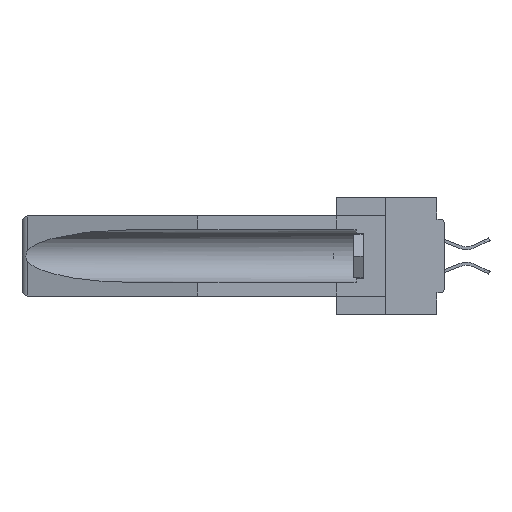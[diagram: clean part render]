
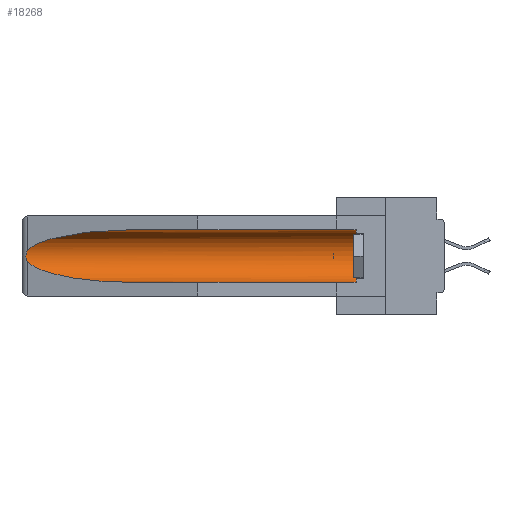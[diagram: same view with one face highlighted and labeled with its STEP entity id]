
A CAD part, left-side view. The second image highlights one B-rep face of the part: STEP entity #18268.
In plain terms, the highlighted cylindrical face has radius 2.857 mm (diameter 5.715 mm), a partial arc.
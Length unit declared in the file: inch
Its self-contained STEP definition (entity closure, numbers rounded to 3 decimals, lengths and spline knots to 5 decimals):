
#1574 =( BOUNDED_CURVE ( )  B_SPLINE_CURVE ( 3, ( #16158, #28046, #19972, #5374 ),
 .UNSPECIFIED., .F., .F. ) 
 B_SPLINE_CURVE_WITH_KNOTS ( ( 4, 4 ),
 ( 4.71239, 6.08839 ),
 .UNSPECIFIED. ) 
 CURVE ( )  GEOMETRIC_REPRESENTATION_ITEM ( )  RATIONAL_B_SPLINE_CURVE ( ( 1., 0.848, 0.848, 1. ) ) 
 REPRESENTATION_ITEM ( '' )  );
#3308 = CARTESIAN_POINT ( 'NONE',  ( 0.26597, 1.5296, -0.19026 ) ) ;
#5374 = CARTESIAN_POINT ( 'NONE',  ( 0.26537, 1.52718, -0.14972 ) ) ;
#6934 = LINE ( 'NONE', #43947, #14084 ) ;
#10229 = CYLINDRICAL_SURFACE ( 'NONE', #19563, 0.1125 ) ;
#10656 = CARTESIAN_POINT ( 'NONE',  ( 0.26537, 1.52718, -0.14972 ) ) ;
#10883 = CARTESIAN_POINT ( 'NONE',  ( 0.25451, 1.48313, -0.24835 ) ) ;
#11092 = CARTESIAN_POINT ( 'NONE',  ( 0.26655, 1.53094, -0.18657 ) ) ;
#12966 = CARTESIAN_POINT ( 'NONE',  ( 0.155, 1.07973, -0.284 ) ) ;
#14084 = VECTOR ( 'NONE', #48096, 39.37008 ) ;
#14113 = EDGE_CURVE ( 'NONE', #47181, #30268, #31578, .T. ) ;
#14117 = CARTESIAN_POINT ( 'NONE',  ( 0.26537, 1.52718, -0.19328 ) ) ;
#16128 = ORIENTED_EDGE ( 'NONE', *, *, #14113, .T. ) ;
#16158 = CARTESIAN_POINT ( 'NONE',  ( 0.155, 1.07973, -0.059 ) ) ;
#17837 = CARTESIAN_POINT ( 'NONE',  ( 0.26537, 1.52718, -0.14972 ) ) ;
#18268 = ADVANCED_FACE ( 'NONE', ( #47509 ), #10229, .F. ) ;
#18936 = VECTOR ( 'NONE', #21263, 39.37008 ) ;
#19563 = AXIS2_PLACEMENT_3D ( 'NONE', #37400, #22460, #33725 ) ;
#19953 = VERTEX_POINT ( 'NONE', #10656 ) ;
#19972 = CARTESIAN_POINT ( 'NONE',  ( 0.25451, 1.48313, -0.09465 ) ) ;
#20417 = CARTESIAN_POINT ( 'NONE',  ( 0.155, 1.07973, -0.059 ) ) ;
#20473 = CARTESIAN_POINT ( 'NONE',  ( 0.155, 0.126, -0.284 ) ) ;
#21263 = DIRECTION ( 'NONE',  ( 0., 1., 0. ) ) ;
#21449 = CARTESIAN_POINT ( 'NONE',  ( 0.26537, 1.52718, -0.19328 ) ) ;
#21588 = CARTESIAN_POINT ( 'NONE',  ( 0.155, -0.30754, -0.284 ) ) ;
#21740 = VERTEX_POINT ( 'NONE', #12966 ) ;
#22326 = CARTESIAN_POINT ( 'NONE',  ( 0.2675, 1.53308, -0.16763 ) ) ;
#22460 = DIRECTION ( 'NONE',  ( 0., 1., 0. ) ) ;
#22610 = EDGE_CURVE ( 'NONE', #37129, #19953, #1574, .T. ) ;
#26129 = CARTESIAN_POINT ( 'NONE',  ( 0.26537, 1.52718, -0.19328 ) ) ;
#26180 = CARTESIAN_POINT ( 'NONE',  ( 0.155, 0.126, -0.1715 ) ) ;
#26446 = CARTESIAN_POINT ( 'NONE',  ( 0.2675, 1.53308, -0.17534 ) ) ;
#28046 = CARTESIAN_POINT ( 'NONE',  ( 0.21114, 1.30732, -0.059 ) ) ;
#28497 = EDGE_CURVE ( 'NONE', #19953, #35295, #41975, .T. ) ;
#29026 = LINE ( 'NONE', #21588, #18936 ) ;
#29615 = CARTESIAN_POINT ( 'NONE',  ( 0.26654, 1.53092, -0.15636 ) ) ;
#29767 = CARTESIAN_POINT ( 'NONE',  ( 0.2673, 1.53269, -0.17917 ) ) ;
#30268 = VERTEX_POINT ( 'NONE', #47377 ) ;
#31578 = CIRCLE ( 'NONE', #34379, 0.1125 ) ;
#32881 = CARTESIAN_POINT ( 'NONE',  ( 0.155, 1.07973, -0.284 ) ) ;
#33725 = DIRECTION ( 'NONE',  ( 0., 0., 1. ) ) ;
#33807 = EDGE_CURVE ( 'NONE', #47181, #21740, #29026, .T. ) ;
#34149 = DIRECTION ( 'NONE',  ( 0., -1., 0. ) ) ;
#34379 = AXIS2_PLACEMENT_3D ( 'NONE', #26180, #34149, #38127 ) ;
#34685 =( BOUNDED_CURVE ( )  B_SPLINE_CURVE ( 3, ( #21449, #10883, #36874, #32881 ),
 .UNSPECIFIED., .F., .F. ) 
 B_SPLINE_CURVE_WITH_KNOTS ( ( 4, 4 ),
 ( 0.1948, 1.5708 ),
 .UNSPECIFIED. ) 
 CURVE ( )  GEOMETRIC_REPRESENTATION_ITEM ( )  RATIONAL_B_SPLINE_CURVE ( ( 1., 0.848, 0.848, 1. ) ) 
 REPRESENTATION_ITEM ( '' )  );
#35182 = EDGE_CURVE ( 'NONE', #30268, #37129, #6934, .T. ) ;
#35295 = VERTEX_POINT ( 'NONE', #14117 ) ;
#35565 = ORIENTED_EDGE ( 'NONE', *, *, #35182, .T. ) ;
#36874 = CARTESIAN_POINT ( 'NONE',  ( 0.21114, 1.30732, -0.284 ) ) ;
#37129 = VERTEX_POINT ( 'NONE', #20417 ) ;
#37400 = CARTESIAN_POINT ( 'NONE',  ( 0.155, -0.30754, -0.1715 ) ) ;
#38127 = DIRECTION ( 'NONE',  ( 0., 0., 1. ) ) ;
#38648 = ORIENTED_EDGE ( 'NONE', *, *, #28497, .T. ) ;
#39947 = EDGE_CURVE ( 'NONE', #35295, #21740, #34685, .T. ) ;
#40312 = EDGE_LOOP ( 'NONE', ( #44161, #38648, #46087, #41166, #16128, #35565 ) ) ;
#41166 = ORIENTED_EDGE ( 'NONE', *, *, #33807, .F. ) ;
#41975 = B_SPLINE_CURVE_WITH_KNOTS ( 'NONE', 3,
 ( #17837, #44376, #29615, #48200, #22326, #26446, #29767, #11092, #3308, #26129 ),
 .UNSPECIFIED., .F., .F.,
 ( 4, 2, 2, 2, 4 ),
 ( 0., 0.00029, 0.00058, 0.00087, 0.00117 ),
 .UNSPECIFIED. ) ;
#43947 = CARTESIAN_POINT ( 'NONE',  ( 0.155, -0.30754, -0.059 ) ) ;
#44161 = ORIENTED_EDGE ( 'NONE', *, *, #22610, .T. ) ;
#44376 = CARTESIAN_POINT ( 'NONE',  ( 0.26597, 1.52961, -0.15275 ) ) ;
#46087 = ORIENTED_EDGE ( 'NONE', *, *, #39947, .T. ) ;
#47181 = VERTEX_POINT ( 'NONE', #20473 ) ;
#47377 = CARTESIAN_POINT ( 'NONE',  ( 0.155, 0.126, -0.059 ) ) ;
#47509 = FACE_OUTER_BOUND ( 'NONE', #40312, .T. ) ;
#48096 = DIRECTION ( 'NONE',  ( 0., 1., 0. ) ) ;
#48200 = CARTESIAN_POINT ( 'NONE',  ( 0.2673, 1.5327, -0.16383 ) ) ;
